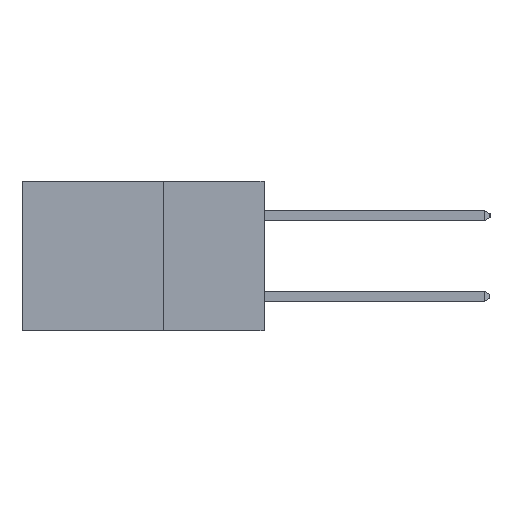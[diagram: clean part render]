
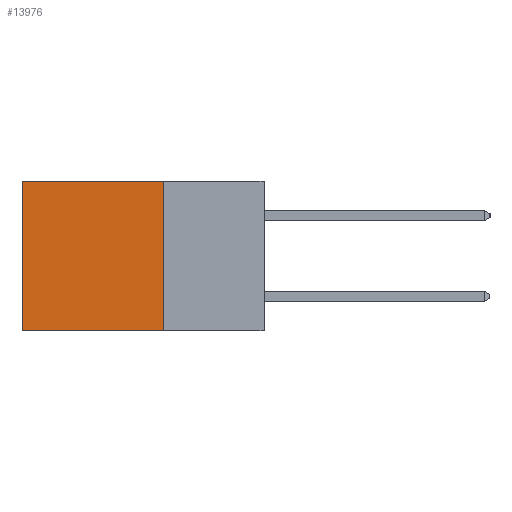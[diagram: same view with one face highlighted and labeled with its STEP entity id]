
A CAD part, left-side view. The second image highlights one B-rep face of the part: STEP entity #13976.
In plain terms, the highlighted planar face has unit normal (-1, 0, 0).
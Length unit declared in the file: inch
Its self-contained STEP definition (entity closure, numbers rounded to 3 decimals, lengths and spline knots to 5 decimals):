
#428 = EDGE_CURVE ( 'NONE', #7230, #2349, #15990, .T. ) ;
#870 = VECTOR ( 'NONE', #12295, 39.37008 ) ;
#1458 = CARTESIAN_POINT ( 'NONE',  ( 0.298, 0.6, -0.37 ) ) ;
#2051 = CARTESIAN_POINT ( 'NONE',  ( 0.298, 0.25, -0.37 ) ) ;
#2349 = VERTEX_POINT ( 'NONE', #17568 ) ;
#2714 = VECTOR ( 'NONE', #15079, 39.37008 ) ;
#3683 = CARTESIAN_POINT ( 'NONE',  ( 0.298, 0.6, 0. ) ) ;
#4703 = CARTESIAN_POINT ( 'NONE',  ( 0.298, 0.25, 0. ) ) ;
#6412 = CARTESIAN_POINT ( 'NONE',  ( 0.298, 0.25, 0. ) ) ;
#6477 = LINE ( 'NONE', #3683, #2714 ) ;
#6674 = VERTEX_POINT ( 'NONE', #2051 ) ;
#7101 = LINE ( 'NONE', #13635, #14239 ) ;
#7230 = VERTEX_POINT ( 'NONE', #4703 ) ;
#7330 = ORIENTED_EDGE ( 'NONE', *, *, #10074, .F. ) ;
#7652 = EDGE_CURVE ( 'NONE', #6674, #8373, #10299, .T. ) ;
#7836 = FACE_OUTER_BOUND ( 'NONE', #17432, .T. ) ;
#7847 = DIRECTION ( 'NONE',  ( 1., 0., 0. ) ) ;
#8373 = VERTEX_POINT ( 'NONE', #1458 ) ;
#9856 = DIRECTION ( 'NONE',  ( 0., 1., 0. ) ) ;
#10074 = EDGE_CURVE ( 'NONE', #7230, #6674, #7101, .T. ) ;
#10299 = LINE ( 'NONE', #16967, #11208 ) ;
#10671 = PLANE ( 'NONE',  #14520 ) ;
#10930 = ORIENTED_EDGE ( 'NONE', *, *, #7652, .F. ) ;
#11208 = VECTOR ( 'NONE', #9856, 39.37008 ) ;
#11936 = ORIENTED_EDGE ( 'NONE', *, *, #14028, .T. ) ;
#12295 = DIRECTION ( 'NONE',  ( 0., 1., 0. ) ) ;
#13635 = CARTESIAN_POINT ( 'NONE',  ( 0.298, 0.25, 0. ) ) ;
#13713 = CARTESIAN_POINT ( 'NONE',  ( 0.298, 0.25, 0. ) ) ;
#13976 = ADVANCED_FACE ( 'NONE', ( #7836 ), #10671, .F. ) ;
#14028 = EDGE_CURVE ( 'NONE', #2349, #8373, #6477, .T. ) ;
#14239 = VECTOR ( 'NONE', #15073, 39.37008 ) ;
#14241 = ORIENTED_EDGE ( 'NONE', *, *, #428, .T. ) ;
#14520 = AXIS2_PLACEMENT_3D ( 'NONE', #6412, #7847, #17809 ) ;
#15073 = DIRECTION ( 'NONE',  ( 0., 0., -1. ) ) ;
#15079 = DIRECTION ( 'NONE',  ( 0., 0., -1. ) ) ;
#15990 = LINE ( 'NONE', #13713, #870 ) ;
#16967 = CARTESIAN_POINT ( 'NONE',  ( 0.298, 0.25, -0.37 ) ) ;
#17432 = EDGE_LOOP ( 'NONE', ( #11936, #10930, #7330, #14241 ) ) ;
#17568 = CARTESIAN_POINT ( 'NONE',  ( 0.298, 0.6, 0. ) ) ;
#17809 = DIRECTION ( 'NONE',  ( 0., 0., -1. ) ) ;
